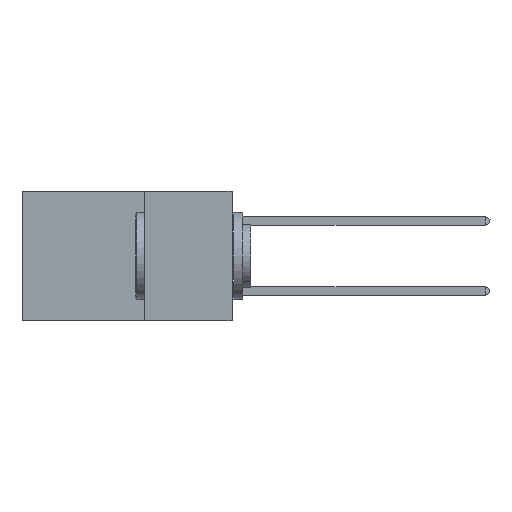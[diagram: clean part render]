
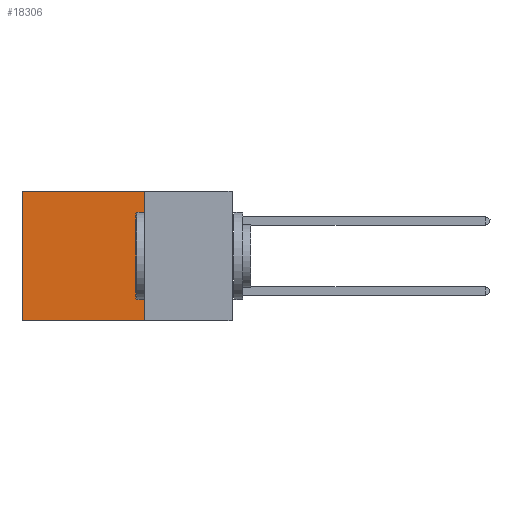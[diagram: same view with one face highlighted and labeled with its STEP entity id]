
A CAD part, left-side view. The second image highlights one B-rep face of the part: STEP entity #18306.
In plain terms, the highlighted planar face has unit normal (-1, 0, 0).
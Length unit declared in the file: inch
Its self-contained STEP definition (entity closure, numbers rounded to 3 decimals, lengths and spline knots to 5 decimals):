
#205 = CARTESIAN_POINT ( 'NONE',  ( 0.2875, 0.25, -0.37 ) ) ;
#737 = EDGE_CURVE ( 'NONE', #37067, #2324, #32427, .T. ) ;
#863 = ORIENTED_EDGE ( 'NONE', *, *, #13811, .T. ) ;
#1126 = DIRECTION ( 'NONE',  ( 0., 1., 0. ) ) ;
#2324 = VERTEX_POINT ( 'NONE', #8748 ) ;
#3128 = DIRECTION ( 'NONE',  ( 0., 1., 0. ) ) ;
#3450 = PLANE ( 'NONE',  #16015 ) ;
#3639 = LINE ( 'NONE', #20468, #18312 ) ;
#8748 = CARTESIAN_POINT ( 'NONE',  ( 0.2875, 0.25, -0.37 ) ) ;
#12629 = CARTESIAN_POINT ( 'NONE',  ( 0.2875, 0.25, 0. ) ) ;
#13811 = EDGE_CURVE ( 'NONE', #37662, #22720, #3639, .T. ) ;
#15269 = DIRECTION ( 'NONE',  ( 0., 0., -1. ) ) ;
#16015 = AXIS2_PLACEMENT_3D ( 'NONE', #17817, #20867, #26759 ) ;
#16720 = VECTOR ( 'NONE', #1126, 39.37008 ) ;
#17817 = CARTESIAN_POINT ( 'NONE',  ( 0.2875, 0.25, 0. ) ) ;
#18306 = ADVANCED_FACE ( 'NONE', ( #23505 ), #3450, .F. ) ;
#18312 = VECTOR ( 'NONE', #15269, 39.37008 ) ;
#19033 = CARTESIAN_POINT ( 'NONE',  ( 0.2875, 0.6, -0.37 ) ) ;
#20405 = ORIENTED_EDGE ( 'NONE', *, *, #26490, .T. ) ;
#20468 = CARTESIAN_POINT ( 'NONE',  ( 0.2875, 0.6, 0. ) ) ;
#20867 = DIRECTION ( 'NONE',  ( 1., 0., 0. ) ) ;
#21367 = ORIENTED_EDGE ( 'NONE', *, *, #737, .F. ) ;
#22720 = VERTEX_POINT ( 'NONE', #19033 ) ;
#23505 = FACE_OUTER_BOUND ( 'NONE', #34741, .T. ) ;
#24547 = LINE ( 'NONE', #27167, #16720 ) ;
#25086 = DIRECTION ( 'NONE',  ( 0., 0., -1. ) ) ;
#26490 = EDGE_CURVE ( 'NONE', #37067, #37662, #24547, .T. ) ;
#26583 = CARTESIAN_POINT ( 'NONE',  ( 0.2875, 0.6, 0. ) ) ;
#26759 = DIRECTION ( 'NONE',  ( 0., 0., -1. ) ) ;
#26873 = CARTESIAN_POINT ( 'NONE',  ( 0.2875, 0.25, 0. ) ) ;
#27167 = CARTESIAN_POINT ( 'NONE',  ( 0.2875, 0.25, 0. ) ) ;
#30731 = EDGE_CURVE ( 'NONE', #2324, #22720, #30812, .T. ) ;
#30812 = LINE ( 'NONE', #205, #36342 ) ;
#32427 = LINE ( 'NONE', #26873, #34307 ) ;
#33188 = ORIENTED_EDGE ( 'NONE', *, *, #30731, .F. ) ;
#34307 = VECTOR ( 'NONE', #25086, 39.37008 ) ;
#34741 = EDGE_LOOP ( 'NONE', ( #863, #33188, #21367, #20405 ) ) ;
#36342 = VECTOR ( 'NONE', #3128, 39.37008 ) ;
#37067 = VERTEX_POINT ( 'NONE', #12629 ) ;
#37662 = VERTEX_POINT ( 'NONE', #26583 ) ;
